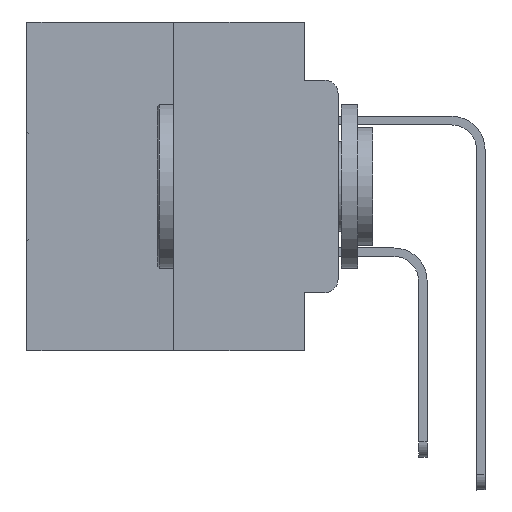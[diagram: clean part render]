
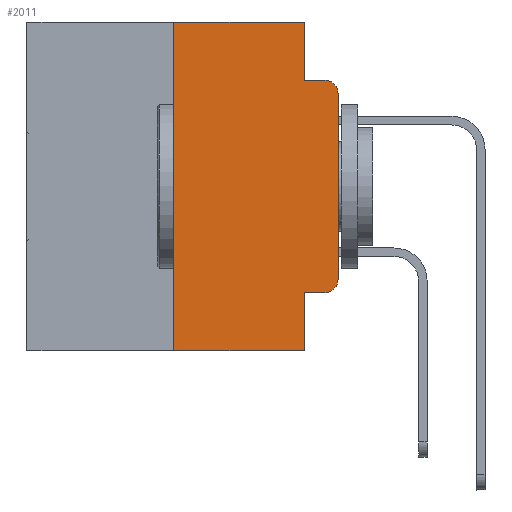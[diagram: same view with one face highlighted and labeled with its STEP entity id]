
A CAD part, left-side view. The second image highlights one B-rep face of the part: STEP entity #2011.
In plain terms, the highlighted planar face has unit normal (-1, 0, 0).
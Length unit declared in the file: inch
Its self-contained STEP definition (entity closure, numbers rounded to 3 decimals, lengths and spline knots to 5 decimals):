
#118 = EDGE_CURVE ( 'NONE', #24830, #12359, #8926, .T. ) ;
#187 = VECTOR ( 'NONE', #11670, 39.37008 ) ;
#1230 = VECTOR ( 'NONE', #2867, 39.37008 ) ;
#1446 = ORIENTED_EDGE ( 'NONE', *, *, #10042, .F. ) ;
#1977 = DIRECTION ( 'NONE',  ( -1., 0., 0. ) ) ;
#2011 = ADVANCED_FACE ( 'NONE', ( #30503 ), #28501, .F. ) ;
#2867 = DIRECTION ( 'NONE',  ( 0., -1., 0. ) ) ;
#3453 = CARTESIAN_POINT ( 'NONE',  ( 0., 0.473, -0.5 ) ) ;
#4962 = AXIS2_PLACEMENT_3D ( 'NONE', #11268, #30899, #16228 ) ;
#6337 = EDGE_CURVE ( 'NONE', #31391, #16012, #6496, .T. ) ;
#6354 = CARTESIAN_POINT ( 'NONE',  ( 0., 0.051, 0. ) ) ;
#6455 = DIRECTION ( 'NONE',  ( 0., 0., -1. ) ) ;
#6496 = LINE ( 'NONE', #3453, #11448 ) ;
#6601 = ORIENTED_EDGE ( 'NONE', *, *, #8445, .F. ) ;
#6759 = ORIENTED_EDGE ( 'NONE', *, *, #6337, .T. ) ;
#7891 = CARTESIAN_POINT ( 'NONE',  ( 0., 0.051, -0.4115 ) ) ;
#7894 = ORIENTED_EDGE ( 'NONE', *, *, #29185, .T. ) ;
#8347 = DIRECTION ( 'NONE',  ( 0., -1., 0. ) ) ;
#8445 = EDGE_CURVE ( 'NONE', #31391, #31794, #10663, .T. ) ;
#8474 = VERTEX_POINT ( 'NONE', #24353 ) ;
#8607 = LINE ( 'NONE', #17535, #1230 ) ;
#8692 = LINE ( 'NONE', #24346, #14355 ) ;
#8846 = CARTESIAN_POINT ( 'NONE',  ( 0., 0., -0.1085 ) ) ;
#8926 = CIRCLE ( 'NONE', #20801, 0.02 ) ;
#9246 = CARTESIAN_POINT ( 'NONE',  ( 0., 0.473, 0. ) ) ;
#9521 = DIRECTION ( 'NONE',  ( 0., 0., 1. ) ) ;
#10042 = EDGE_CURVE ( 'NONE', #31348, #16012, #8692, .T. ) ;
#10663 = LINE ( 'NONE', #26738, #15667 ) ;
#11064 = EDGE_CURVE ( 'NONE', #18011, #8474, #23589, .T. ) ;
#11148 = CARTESIAN_POINT ( 'NONE',  ( 0., 0.25, -0.5 ) ) ;
#11268 = CARTESIAN_POINT ( 'NONE',  ( 0., 0.473, 0. ) ) ;
#11448 = VECTOR ( 'NONE', #8347, 39.37008 ) ;
#11670 = DIRECTION ( 'NONE',  ( 0., -1., 0. ) ) ;
#11977 = VECTOR ( 'NONE', #27545, 39.37008 ) ;
#12359 = VERTEX_POINT ( 'NONE', #21322 ) ;
#13050 = CARTESIAN_POINT ( 'NONE',  ( 0., 0., 0. ) ) ;
#13337 = ORIENTED_EDGE ( 'NONE', *, *, #30382, .T. ) ;
#14355 = VECTOR ( 'NONE', #29264, 39.37008 ) ;
#14753 = VECTOR ( 'NONE', #30250, 39.37008 ) ;
#14948 = EDGE_CURVE ( 'NONE', #8474, #27994, #8607, .T. ) ;
#15667 = VECTOR ( 'NONE', #9521, 39.37008 ) ;
#16012 = VERTEX_POINT ( 'NONE', #31638 ) ;
#16228 = DIRECTION ( 'NONE',  ( 0., 0., -1. ) ) ;
#16741 = CARTESIAN_POINT ( 'NONE',  ( 0., 0.02, -0.1085 ) ) ;
#17076 = EDGE_CURVE ( 'NONE', #26324, #27994, #20367, .T. ) ;
#17086 = ORIENTED_EDGE ( 'NONE', *, *, #118, .T. ) ;
#17535 = CARTESIAN_POINT ( 'NONE',  ( 0., 0.051, -0.0885 ) ) ;
#18011 = VERTEX_POINT ( 'NONE', #20049 ) ;
#18281 = AXIS2_PLACEMENT_3D ( 'NONE', #16741, #1977, #19250 ) ;
#18525 = ORIENTED_EDGE ( 'NONE', *, *, #17076, .T. ) ;
#18528 = CARTESIAN_POINT ( 'NONE',  ( 0., 0.02, -0.3915 ) ) ;
#19250 = DIRECTION ( 'NONE',  ( 0., 0., -1. ) ) ;
#19862 = LINE ( 'NONE', #9246, #187 ) ;
#20049 = CARTESIAN_POINT ( 'NONE',  ( 0., 0.051, 0. ) ) ;
#20136 = LINE ( 'NONE', #7891, #11977 ) ;
#20367 = CIRCLE ( 'NONE', #18281, 0.02 ) ;
#20755 = CARTESIAN_POINT ( 'NONE',  ( 0., 0.051, -0.4115 ) ) ;
#20801 = AXIS2_PLACEMENT_3D ( 'NONE', #18528, #23118, #28812 ) ;
#21322 = CARTESIAN_POINT ( 'NONE',  ( 0., 0., -0.3915 ) ) ;
#21355 = LINE ( 'NONE', #13050, #14753 ) ;
#21704 = EDGE_LOOP ( 'NONE', ( #7894, #18525, #23827, #23851, #22451, #6601, #6759, #1446, #13337, #17086 ) ) ;
#22044 = VECTOR ( 'NONE', #6455, 39.37008 ) ;
#22451 = ORIENTED_EDGE ( 'NONE', *, *, #28822, .F. ) ;
#22766 = CARTESIAN_POINT ( 'NONE',  ( 0., 0.02, -0.4115 ) ) ;
#23118 = DIRECTION ( 'NONE',  ( -1., 0., 0. ) ) ;
#23589 = LINE ( 'NONE', #6354, #22044 ) ;
#23827 = ORIENTED_EDGE ( 'NONE', *, *, #14948, .F. ) ;
#23851 = ORIENTED_EDGE ( 'NONE', *, *, #11064, .F. ) ;
#24346 = CARTESIAN_POINT ( 'NONE',  ( 0., 0.051, 0. ) ) ;
#24353 = CARTESIAN_POINT ( 'NONE',  ( 0., 0.051, -0.0885 ) ) ;
#24830 = VERTEX_POINT ( 'NONE', #22766 ) ;
#25452 = CARTESIAN_POINT ( 'NONE',  ( 0., 0.25, 0. ) ) ;
#26324 = VERTEX_POINT ( 'NONE', #8846 ) ;
#26738 = CARTESIAN_POINT ( 'NONE',  ( 0., 0.25, 0. ) ) ;
#27545 = DIRECTION ( 'NONE',  ( 0., -1., 0. ) ) ;
#27577 = CARTESIAN_POINT ( 'NONE',  ( 0., 0.02, -0.0885 ) ) ;
#27994 = VERTEX_POINT ( 'NONE', #27577 ) ;
#28501 = PLANE ( 'NONE',  #4962 ) ;
#28812 = DIRECTION ( 'NONE',  ( 0., 0., -1. ) ) ;
#28822 = EDGE_CURVE ( 'NONE', #31794, #18011, #19862, .T. ) ;
#29185 = EDGE_CURVE ( 'NONE', #12359, #26324, #21355, .T. ) ;
#29264 = DIRECTION ( 'NONE',  ( 0., 0., -1. ) ) ;
#30250 = DIRECTION ( 'NONE',  ( 0., 0., 1. ) ) ;
#30382 = EDGE_CURVE ( 'NONE', #31348, #24830, #20136, .T. ) ;
#30503 = FACE_OUTER_BOUND ( 'NONE', #21704, .T. ) ;
#30899 = DIRECTION ( 'NONE',  ( 1., 0., 0. ) ) ;
#31348 = VERTEX_POINT ( 'NONE', #20755 ) ;
#31391 = VERTEX_POINT ( 'NONE', #11148 ) ;
#31638 = CARTESIAN_POINT ( 'NONE',  ( 0., 0.051, -0.5 ) ) ;
#31794 = VERTEX_POINT ( 'NONE', #25452 ) ;
